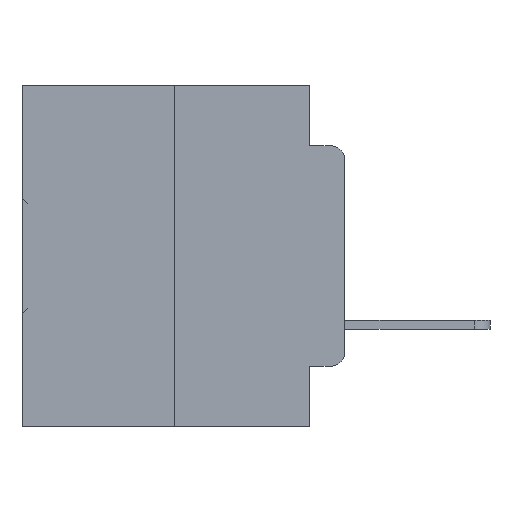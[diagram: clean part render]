
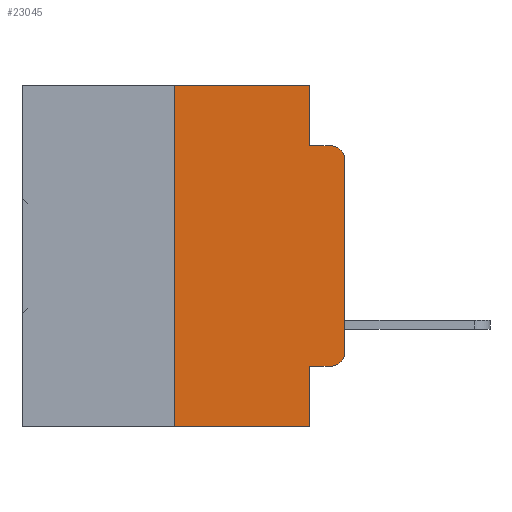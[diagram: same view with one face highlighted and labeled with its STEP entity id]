
A CAD part, left-side view. The second image highlights one B-rep face of the part: STEP entity #23045.
In plain terms, the highlighted planar face has unit normal (-1, 0, 0).
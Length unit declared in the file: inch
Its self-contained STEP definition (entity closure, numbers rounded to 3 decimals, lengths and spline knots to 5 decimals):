
#609 = ORIENTED_EDGE ( 'NONE', *, *, #18482, .T. ) ;
#895 = ORIENTED_EDGE ( 'NONE', *, *, #20502, .T. ) ;
#940 = CARTESIAN_POINT ( 'NONE',  ( 0., 0., -0.3915 ) ) ;
#1047 = ORIENTED_EDGE ( 'NONE', *, *, #26462, .F. ) ;
#1226 = DIRECTION ( 'NONE',  ( 0., 0., 1. ) ) ;
#1289 = VERTEX_POINT ( 'NONE', #13846 ) ;
#1334 = DIRECTION ( 'NONE',  ( 0., -1., 0. ) ) ;
#1401 = ORIENTED_EDGE ( 'NONE', *, *, #25942, .F. ) ;
#1570 = LINE ( 'NONE', #27497, #7249 ) ;
#1618 = ORIENTED_EDGE ( 'NONE', *, *, #2529, .F. ) ;
#1926 = DIRECTION ( 'NONE',  ( 0., 0., -1. ) ) ;
#2254 = CARTESIAN_POINT ( 'NONE',  ( 0., 0.02, -0.4115 ) ) ;
#2529 = EDGE_CURVE ( 'NONE', #4243, #23506, #22020, .T. ) ;
#3265 = LINE ( 'NONE', #33989, #11540 ) ;
#3554 = ORIENTED_EDGE ( 'NONE', *, *, #32188, .F. ) ;
#4100 = AXIS2_PLACEMENT_3D ( 'NONE', #13445, #16174, #34771 ) ;
#4243 = VERTEX_POINT ( 'NONE', #16142 ) ;
#4293 = VERTEX_POINT ( 'NONE', #18634 ) ;
#4515 = VERTEX_POINT ( 'NONE', #940 ) ;
#4544 = CARTESIAN_POINT ( 'NONE',  ( 0., 0.051, -0.5 ) ) ;
#4547 = VERTEX_POINT ( 'NONE', #6689 ) ;
#5118 = PLANE ( 'NONE',  #4100 ) ;
#5260 = CARTESIAN_POINT ( 'NONE',  ( 0., 0.473, -0.5 ) ) ;
#5435 = AXIS2_PLACEMENT_3D ( 'NONE', #11308, #30112, #14048 ) ;
#6204 = CARTESIAN_POINT ( 'NONE',  ( 0., 0., -0.1085 ) ) ;
#6689 = CARTESIAN_POINT ( 'NONE',  ( 0., 0.25, -0.5 ) ) ;
#7011 = DIRECTION ( 'NONE',  ( -1., 0., 0. ) ) ;
#7055 = EDGE_CURVE ( 'NONE', #18071, #4515, #15915, .T. ) ;
#7074 = ORIENTED_EDGE ( 'NONE', *, *, #22518, .T. ) ;
#7249 = VECTOR ( 'NONE', #32863, 39.37008 ) ;
#7797 = ORIENTED_EDGE ( 'NONE', *, *, #8171, .F. ) ;
#8058 = DIRECTION ( 'NONE',  ( 0., -1., 0. ) ) ;
#8171 = EDGE_CURVE ( 'NONE', #23328, #30181, #32625, .T. ) ;
#9630 = VECTOR ( 'NONE', #1226, 39.37008 ) ;
#10297 = ORIENTED_EDGE ( 'NONE', *, *, #26377, .T. ) ;
#10436 = ORIENTED_EDGE ( 'NONE', *, *, #7055, .T. ) ;
#11221 = VECTOR ( 'NONE', #1926, 39.37008 ) ;
#11308 = CARTESIAN_POINT ( 'NONE',  ( 0., 0.02, -0.1085 ) ) ;
#11540 = VECTOR ( 'NONE', #28774, 39.37008 ) ;
#11896 = CIRCLE ( 'NONE', #5435, 0.02 ) ;
#12309 = VECTOR ( 'NONE', #1334, 39.37008 ) ;
#12398 = CARTESIAN_POINT ( 'NONE',  ( 0., 0.051, -0.4115 ) ) ;
#13445 = CARTESIAN_POINT ( 'NONE',  ( 0., 0.473, 0. ) ) ;
#13846 = CARTESIAN_POINT ( 'NONE',  ( 0., 0.051, -0.0885 ) ) ;
#14048 = DIRECTION ( 'NONE',  ( 0., 0., -1. ) ) ;
#14880 = VECTOR ( 'NONE', #19348, 39.37008 ) ;
#15418 = CARTESIAN_POINT ( 'NONE',  ( 0., 0.051, 0. ) ) ;
#15915 = CIRCLE ( 'NONE', #27396, 0.02 ) ;
#16142 = CARTESIAN_POINT ( 'NONE',  ( 0., 0.25, 0. ) ) ;
#16174 = DIRECTION ( 'NONE',  ( 1., 0., 0. ) ) ;
#16833 = LINE ( 'NONE', #5260, #23167 ) ;
#17790 = LINE ( 'NONE', #12398, #12309 ) ;
#18071 = VERTEX_POINT ( 'NONE', #2254 ) ;
#18482 = EDGE_CURVE ( 'NONE', #4515, #29291, #24139, .T. ) ;
#18634 = CARTESIAN_POINT ( 'NONE',  ( 0., 0.02, -0.0885 ) ) ;
#19348 = DIRECTION ( 'NONE',  ( 0., -1., 0. ) ) ;
#20378 = CARTESIAN_POINT ( 'NONE',  ( 0., 0., 0. ) ) ;
#20502 = EDGE_CURVE ( 'NONE', #29291, #4293, #11896, .T. ) ;
#22020 = LINE ( 'NONE', #34384, #14880 ) ;
#22518 = EDGE_CURVE ( 'NONE', #4547, #30181, #16833, .T. ) ;
#22716 = CARTESIAN_POINT ( 'NONE',  ( 0., 0.051, -0.4115 ) ) ;
#23045 = ADVANCED_FACE ( 'NONE', ( #33852 ), #5118, .F. ) ;
#23167 = VECTOR ( 'NONE', #8058, 39.37008 ) ;
#23322 = CARTESIAN_POINT ( 'NONE',  ( 0., 0.02, -0.3915 ) ) ;
#23328 = VERTEX_POINT ( 'NONE', #22716 ) ;
#23506 = VERTEX_POINT ( 'NONE', #15418 ) ;
#23633 = CARTESIAN_POINT ( 'NONE',  ( 0., 0.051, -0.0885 ) ) ;
#24139 = LINE ( 'NONE', #20378, #9630 ) ;
#25942 = EDGE_CURVE ( 'NONE', #23506, #1289, #3265, .T. ) ;
#26042 = DIRECTION ( 'NONE',  ( 0., 0., -1. ) ) ;
#26319 = DIRECTION ( 'NONE',  ( 0., -1., 0. ) ) ;
#26377 = EDGE_CURVE ( 'NONE', #23328, #18071, #17790, .T. ) ;
#26462 = EDGE_CURVE ( 'NONE', #1289, #4293, #28721, .T. ) ;
#27396 = AXIS2_PLACEMENT_3D ( 'NONE', #23322, #7011, #26042 ) ;
#27497 = CARTESIAN_POINT ( 'NONE',  ( 0., 0.25, 0. ) ) ;
#27886 = VECTOR ( 'NONE', #26319, 39.37008 ) ;
#28721 = LINE ( 'NONE', #23633, #27886 ) ;
#28774 = DIRECTION ( 'NONE',  ( 0., 0., -1. ) ) ;
#29291 = VERTEX_POINT ( 'NONE', #6204 ) ;
#30112 = DIRECTION ( 'NONE',  ( -1., 0., 0. ) ) ;
#30181 = VERTEX_POINT ( 'NONE', #4544 ) ;
#31700 = CARTESIAN_POINT ( 'NONE',  ( 0., 0.051, 0. ) ) ;
#32188 = EDGE_CURVE ( 'NONE', #4547, #4243, #1570, .T. ) ;
#32625 = LINE ( 'NONE', #31700, #11221 ) ;
#32863 = DIRECTION ( 'NONE',  ( 0., 0., 1. ) ) ;
#33852 = FACE_OUTER_BOUND ( 'NONE', #34853, .T. ) ;
#33989 = CARTESIAN_POINT ( 'NONE',  ( 0., 0.051, 0. ) ) ;
#34384 = CARTESIAN_POINT ( 'NONE',  ( 0., 0.473, 0. ) ) ;
#34771 = DIRECTION ( 'NONE',  ( 0., 0., -1. ) ) ;
#34853 = EDGE_LOOP ( 'NONE', ( #609, #895, #1047, #1401, #1618, #3554, #7074, #7797, #10297, #10436 ) ) ;
